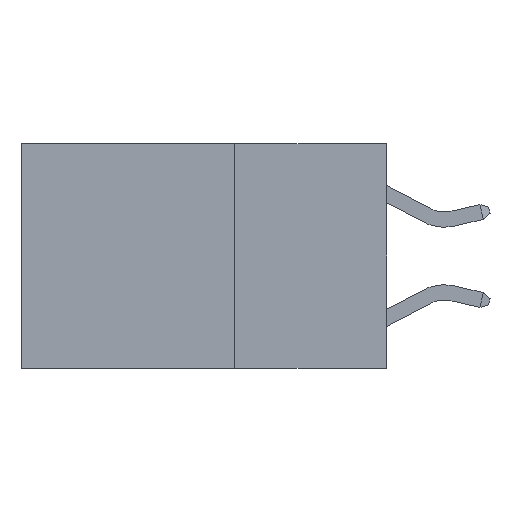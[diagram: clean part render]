
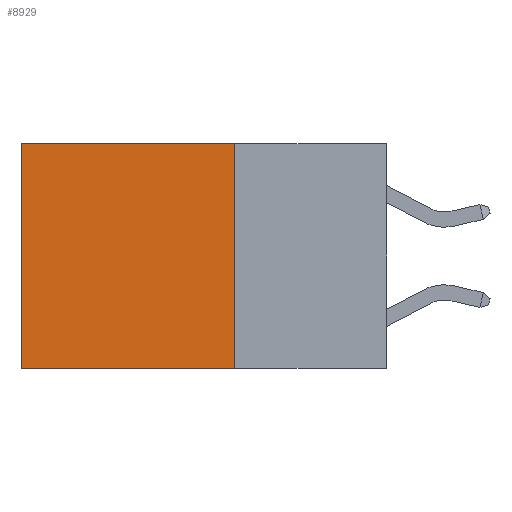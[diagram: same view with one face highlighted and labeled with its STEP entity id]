
A CAD part, left-side view. The second image highlights one B-rep face of the part: STEP entity #8929.
In plain terms, the highlighted planar face has unit normal (-1, 0, 0).
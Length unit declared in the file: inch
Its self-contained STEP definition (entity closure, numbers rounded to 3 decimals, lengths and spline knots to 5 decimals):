
#447 = EDGE_CURVE ( 'NONE', #8023, #5330, #11981, .T. ) ;
#538 = VECTOR ( 'NONE', #899, 39.37008 ) ;
#899 = DIRECTION ( 'NONE',  ( 0., 1., 0. ) ) ;
#1102 = DIRECTION ( 'NONE',  ( 0., 0., -1. ) ) ;
#1274 = CARTESIAN_POINT ( 'NONE',  ( 0.2625, 0.25, 0. ) ) ;
#1592 = CARTESIAN_POINT ( 'NONE',  ( 0.2625, 0.25, 0. ) ) ;
#1817 = PLANE ( 'NONE',  #7710 ) ;
#1829 = CARTESIAN_POINT ( 'NONE',  ( 0.2625, 0.25, 0. ) ) ;
#3423 = DIRECTION ( 'NONE',  ( 1., 0., 0. ) ) ;
#3478 = VERTEX_POINT ( 'NONE', #7484 ) ;
#3606 = EDGE_CURVE ( 'NONE', #8496, #3478, #9629, .T. ) ;
#3917 = CARTESIAN_POINT ( 'NONE',  ( 0.2625, 0.6, 0. ) ) ;
#4172 = ORIENTED_EDGE ( 'NONE', *, *, #10655, .F. ) ;
#5126 = ORIENTED_EDGE ( 'NONE', *, *, #6931, .T. ) ;
#5330 = VERTEX_POINT ( 'NONE', #10846 ) ;
#5342 = DIRECTION ( 'NONE',  ( 0., 1., 0. ) ) ;
#5527 = ORIENTED_EDGE ( 'NONE', *, *, #3606, .T. ) ;
#6358 = EDGE_LOOP ( 'NONE', ( #5527, #4172, #10464, #5126 ) ) ;
#6488 = DIRECTION ( 'NONE',  ( 0., 0., -1. ) ) ;
#6931 = EDGE_CURVE ( 'NONE', #8023, #8496, #10988, .T. ) ;
#7253 = VECTOR ( 'NONE', #1102, 39.37008 ) ;
#7484 = CARTESIAN_POINT ( 'NONE',  ( 0.2625, 0.6, -0.37 ) ) ;
#7696 = CARTESIAN_POINT ( 'NONE',  ( 0.2625, 0.6, 0. ) ) ;
#7710 = AXIS2_PLACEMENT_3D ( 'NONE', #11725, #3423, #10837 ) ;
#8023 = VERTEX_POINT ( 'NONE', #1274 ) ;
#8266 = FACE_OUTER_BOUND ( 'NONE', #6358, .T. ) ;
#8496 = VERTEX_POINT ( 'NONE', #3917 ) ;
#8804 = VECTOR ( 'NONE', #6488, 39.37008 ) ;
#8929 = ADVANCED_FACE ( 'NONE', ( #8266 ), #1817, .F. ) ;
#9487 = LINE ( 'NONE', #10154, #538 ) ;
#9629 = LINE ( 'NONE', #7696, #7253 ) ;
#10154 = CARTESIAN_POINT ( 'NONE',  ( 0.2625, 0.25, -0.37 ) ) ;
#10464 = ORIENTED_EDGE ( 'NONE', *, *, #447, .F. ) ;
#10655 = EDGE_CURVE ( 'NONE', #5330, #3478, #9487, .T. ) ;
#10837 = DIRECTION ( 'NONE',  ( 0., 0., -1. ) ) ;
#10846 = CARTESIAN_POINT ( 'NONE',  ( 0.2625, 0.25, -0.37 ) ) ;
#10988 = LINE ( 'NONE', #1592, #11017 ) ;
#11017 = VECTOR ( 'NONE', #5342, 39.37008 ) ;
#11725 = CARTESIAN_POINT ( 'NONE',  ( 0.2625, 0.25, 0. ) ) ;
#11981 = LINE ( 'NONE', #1829, #8804 ) ;
